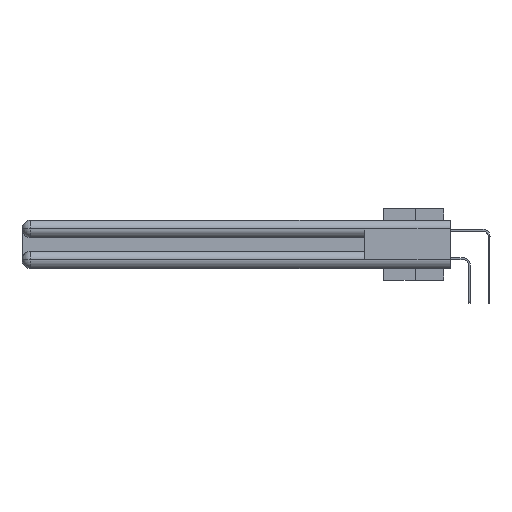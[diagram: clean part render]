
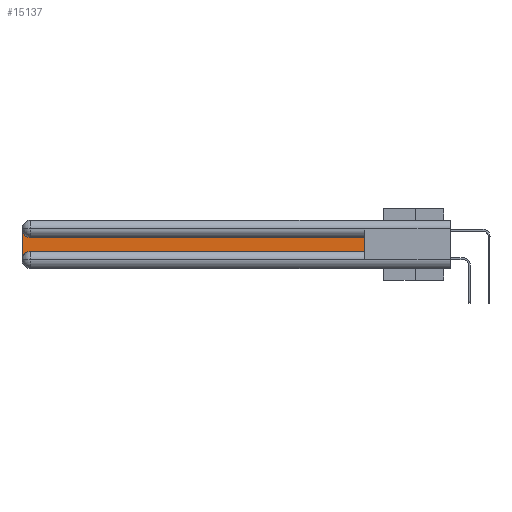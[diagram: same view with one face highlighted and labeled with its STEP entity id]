
A CAD part, left-side view. The second image highlights one B-rep face of the part: STEP entity #15137.
In plain terms, the highlighted planar face has unit normal (-1, 0, 0).
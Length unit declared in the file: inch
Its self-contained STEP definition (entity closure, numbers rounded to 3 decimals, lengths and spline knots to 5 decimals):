
#146 = CARTESIAN_POINT ( 'NONE',  ( 0.075, 2.94, -0.1225 ) ) ;
#225 = CARTESIAN_POINT ( 'NONE',  ( 0.075, 2.94, -0.2175 ) ) ;
#268 = LINE ( 'NONE', #10424, #29120 ) ;
#1090 = CARTESIAN_POINT ( 'NONE',  ( 0.075, 0.6, -0.2175 ) ) ;
#2464 = CARTESIAN_POINT ( 'NONE',  ( 0.075, 3., -0.1225 ) ) ;
#3843 = DIRECTION ( 'NONE',  ( 1., 0., 0. ) ) ;
#3923 = CARTESIAN_POINT ( 'NONE',  ( 0.075, 0.6, -0.2175 ) ) ;
#3945 = VECTOR ( 'NONE', #13597, 39.37008 ) ;
#5234 = VECTOR ( 'NONE', #29238, 39.37008 ) ;
#5257 = EDGE_CURVE ( 'NONE', #14421, #32181, #268, .T. ) ;
#5563 = AXIS2_PLACEMENT_3D ( 'NONE', #21539, #3843, #23731 ) ;
#6711 = ORIENTED_EDGE ( 'NONE', *, *, #16215, .T. ) ;
#7446 = DIRECTION ( 'NONE',  ( 0., 0., -1. ) ) ;
#7529 = ORIENTED_EDGE ( 'NONE', *, *, #19034, .T. ) ;
#8963 = ORIENTED_EDGE ( 'NONE', *, *, #20275, .T. ) ;
#9859 = VERTEX_POINT ( 'NONE', #19148 ) ;
#10424 = CARTESIAN_POINT ( 'NONE',  ( 0.075, 3., -0.2175 ) ) ;
#10587 = VECTOR ( 'NONE', #26266, 39.37008 ) ;
#10620 = CARTESIAN_POINT ( 'NONE',  ( 0.075, 3., -0.2775 ) ) ;
#10823 = CARTESIAN_POINT ( 'NONE',  ( 0.075, 0.6, -0.1225 ) ) ;
#11230 = VERTEX_POINT ( 'NONE', #225 ) ;
#11251 = EDGE_LOOP ( 'NONE', ( #26119, #6711, #31046, #7529, #8963, #27952 ) ) ;
#11305 = CARTESIAN_POINT ( 'NONE',  ( 0.075, 2.94, -0.0625 ) ) ;
#13597 = DIRECTION ( 'NONE',  ( 0., 1., 0. ) ) ;
#14187 = DIRECTION ( 'NONE',  ( 0., 0., -1. ) ) ;
#14421 = VERTEX_POINT ( 'NONE', #31958 ) ;
#15047 = LINE ( 'NONE', #3923, #5234 ) ;
#15137 = ADVANCED_FACE ( 'NONE', ( #16263 ), #30012, .F. ) ;
#15311 = LINE ( 'NONE', #1090, #10587 ) ;
#16215 = EDGE_CURVE ( 'NONE', #22021, #14421, #16598, .T. ) ;
#16263 = FACE_OUTER_BOUND ( 'NONE', #11251, .T. ) ;
#16598 = CIRCLE ( 'NONE', #18454, 0.06 ) ;
#17152 = AXIS2_PLACEMENT_3D ( 'NONE', #2464, #27114, #7446 ) ;
#17356 = CARTESIAN_POINT ( 'NONE',  ( 0.075, 0.6, -0.1225 ) ) ;
#18454 = AXIS2_PLACEMENT_3D ( 'NONE', #11305, #19050, #14187 ) ;
#19034 = EDGE_CURVE ( 'NONE', #32181, #11230, #24324, .T. ) ;
#19050 = DIRECTION ( 'NONE',  ( 1., 0., 0. ) ) ;
#19148 = CARTESIAN_POINT ( 'NONE',  ( 0.075, 0.6, -0.2175 ) ) ;
#20275 = EDGE_CURVE ( 'NONE', #11230, #9859, #15311, .T. ) ;
#21539 = CARTESIAN_POINT ( 'NONE',  ( 0.075, 2.94, -0.2775 ) ) ;
#22021 = VERTEX_POINT ( 'NONE', #146 ) ;
#22323 = LINE ( 'NONE', #10823, #3945 ) ;
#23731 = DIRECTION ( 'NONE',  ( 0., 0., -1. ) ) ;
#23834 = VERTEX_POINT ( 'NONE', #17356 ) ;
#24324 = CIRCLE ( 'NONE', #5563, 0.06 ) ;
#26119 = ORIENTED_EDGE ( 'NONE', *, *, #29116, .T. ) ;
#26266 = DIRECTION ( 'NONE',  ( 0., -1., 0. ) ) ;
#27114 = DIRECTION ( 'NONE',  ( 1., 0., 0. ) ) ;
#27366 = EDGE_CURVE ( 'NONE', #9859, #23834, #15047, .T. ) ;
#27952 = ORIENTED_EDGE ( 'NONE', *, *, #27366, .T. ) ;
#29116 = EDGE_CURVE ( 'NONE', #23834, #22021, #22323, .T. ) ;
#29120 = VECTOR ( 'NONE', #29940, 39.37008 ) ;
#29238 = DIRECTION ( 'NONE',  ( 0., 0., 1. ) ) ;
#29940 = DIRECTION ( 'NONE',  ( 0., 0., -1. ) ) ;
#30012 = PLANE ( 'NONE',  #17152 ) ;
#31046 = ORIENTED_EDGE ( 'NONE', *, *, #5257, .T. ) ;
#31958 = CARTESIAN_POINT ( 'NONE',  ( 0.075, 3., -0.0625 ) ) ;
#32181 = VERTEX_POINT ( 'NONE', #10620 ) ;
